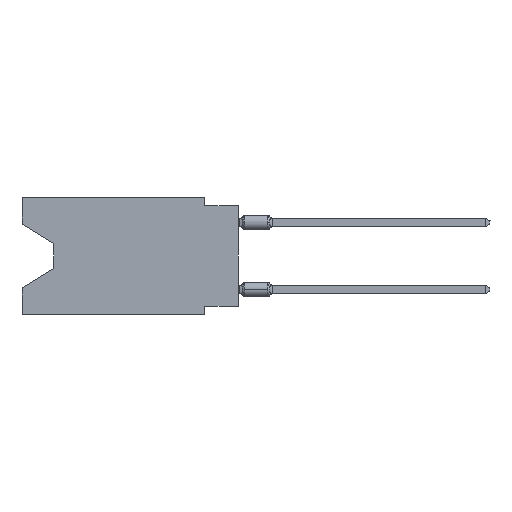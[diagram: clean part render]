
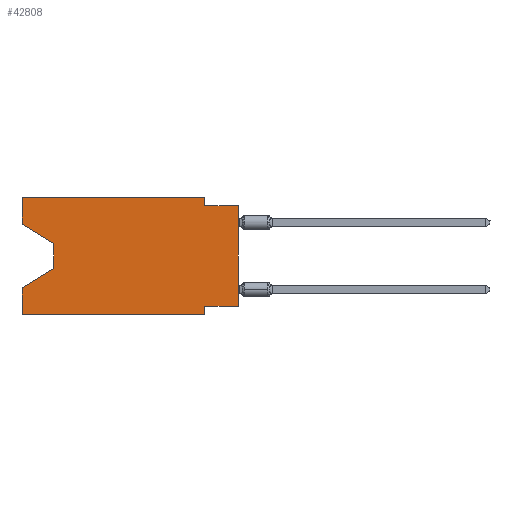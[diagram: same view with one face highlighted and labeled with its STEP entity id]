
A CAD part, left-side view. The second image highlights one B-rep face of the part: STEP entity #42808.
In plain terms, the highlighted planar face has unit normal (-1, 0, 0).
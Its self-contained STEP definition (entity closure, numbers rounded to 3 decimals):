
#393 = VECTOR ( 'NONE', #52997, 1000. ) ;
#806 = VERTEX_POINT ( 'NONE', #63319 ) ;
#818 = DIRECTION ( 'NONE',  ( 0., -1., 0. ) ) ;
#3317 = CARTESIAN_POINT ( 'NONE',  ( 0., 16.383, 0. ) ) ;
#4105 = EDGE_CURVE ( 'NONE', #806, #37848, #15259, .T. ) ;
#4121 = VERTEX_POINT ( 'NONE', #20977 ) ;
#6021 = CARTESIAN_POINT ( 'NONE',  ( 0., 2.54, -8.89 ) ) ;
#6137 = EDGE_CURVE ( 'NONE', #69450, #10985, #16919, .T. ) ;
#6158 = PLANE ( 'NONE',  #10852 ) ;
#6751 = VECTOR ( 'NONE', #17231, 1000. ) ;
#7241 = DIRECTION ( 'NONE',  ( 0., 0.855, -0.519 ) ) ;
#9700 = CARTESIAN_POINT ( 'NONE',  ( 0., 2.54, -0.635 ) ) ;
#9800 = DIRECTION ( 'NONE',  ( 0., -1., 0. ) ) ;
#10821 = VECTOR ( 'NONE', #56934, 1000. ) ;
#10852 = AXIS2_PLACEMENT_3D ( 'NONE', #21896, #70353, #21548 ) ;
#10985 = VERTEX_POINT ( 'NONE', #53490 ) ;
#12302 = EDGE_CURVE ( 'NONE', #4121, #63209, #33869, .T. ) ;
#13230 = VECTOR ( 'NONE', #44570, 1000. ) ;
#13774 = LINE ( 'NONE', #46919, #10821 ) ;
#13959 = VERTEX_POINT ( 'NONE', #39909 ) ;
#14126 = VERTEX_POINT ( 'NONE', #68708 ) ;
#14382 = EDGE_CURVE ( 'NONE', #14126, #55716, #55510, .T. ) ;
#15259 = LINE ( 'NONE', #42722, #27439 ) ;
#16164 = LINE ( 'NONE', #59671, #6751 ) ;
#16919 = LINE ( 'NONE', #38690, #42209 ) ;
#17231 = DIRECTION ( 'NONE',  ( 0., 0., -1. ) ) ;
#20310 = CARTESIAN_POINT ( 'NONE',  ( 0., 2.54, 0. ) ) ;
#20862 = CARTESIAN_POINT ( 'NONE',  ( 0., 16.383, 0. ) ) ;
#20977 = CARTESIAN_POINT ( 'NONE',  ( 0., 2.54, -8.255 ) ) ;
#21548 = DIRECTION ( 'NONE',  ( 0., 0., -1. ) ) ;
#21896 = CARTESIAN_POINT ( 'NONE',  ( 0., 16.383, 0. ) ) ;
#22437 = ORIENTED_EDGE ( 'NONE', *, *, #58329, .T. ) ;
#22937 = ORIENTED_EDGE ( 'NONE', *, *, #55519, .F. ) ;
#23330 = CARTESIAN_POINT ( 'NONE',  ( 0., 13.97, -5.385 ) ) ;
#23611 = ORIENTED_EDGE ( 'NONE', *, *, #39152, .F. ) ;
#26426 = EDGE_CURVE ( 'NONE', #37848, #55716, #40421, .T. ) ;
#26533 = FACE_OUTER_BOUND ( 'NONE', #32036, .T. ) ;
#27054 = DIRECTION ( 'NONE',  ( 0., 0., -1. ) ) ;
#27439 = VECTOR ( 'NONE', #27054, 1000. ) ;
#27983 = LINE ( 'NONE', #43311, #67640 ) ;
#28960 = ORIENTED_EDGE ( 'NONE', *, *, #26426, .T. ) ;
#31087 = EDGE_CURVE ( 'NONE', #13959, #806, #68355, .T. ) ;
#32036 = EDGE_LOOP ( 'NONE', ( #70329, #40375, #28960, #38474, #22437, #48964, #60519, #46093, #22937, #23611, #59856, #41739 ) ) ;
#33869 = LINE ( 'NONE', #6021, #13230 ) ;
#33968 = VECTOR ( 'NONE', #57380, 1000. ) ;
#35635 = LINE ( 'NONE', #47025, #33968 ) ;
#36208 = EDGE_CURVE ( 'NONE', #13959, #60650, #35635, .T. ) ;
#36211 = LINE ( 'NONE', #37276, #50064 ) ;
#36373 = VECTOR ( 'NONE', #7241, 1000. ) ;
#37276 = CARTESIAN_POINT ( 'NONE',  ( 0., 0., -8.255 ) ) ;
#37848 = VERTEX_POINT ( 'NONE', #43271 ) ;
#38474 = ORIENTED_EDGE ( 'NONE', *, *, #14382, .F. ) ;
#38690 = CARTESIAN_POINT ( 'NONE',  ( 0., 0., 0. ) ) ;
#39152 = EDGE_CURVE ( 'NONE', #65937, #67887, #16164, .T. ) ;
#39909 = CARTESIAN_POINT ( 'NONE',  ( 0., 16.383, -2.038 ) ) ;
#40375 = ORIENTED_EDGE ( 'NONE', *, *, #4105, .T. ) ;
#40421 = LINE ( 'NONE', #23330, #36373 ) ;
#41035 = VECTOR ( 'NONE', #9800, 1000. ) ;
#41739 = ORIENTED_EDGE ( 'NONE', *, *, #36208, .F. ) ;
#42209 = VECTOR ( 'NONE', #54005, 1000. ) ;
#42265 = DIRECTION ( 'NONE',  ( 0., 1., 0. ) ) ;
#42722 = CARTESIAN_POINT ( 'NONE',  ( 0., 13.97, -3.505 ) ) ;
#42808 = ADVANCED_FACE ( 'NONE', ( #26533 ), #6158, .F. ) ;
#43271 = CARTESIAN_POINT ( 'NONE',  ( 0., 13.97, -5.385 ) ) ;
#43311 = CARTESIAN_POINT ( 'NONE',  ( 0., 0., -0.635 ) ) ;
#43753 = CARTESIAN_POINT ( 'NONE',  ( 0., 16.383, 0. ) ) ;
#44570 = DIRECTION ( 'NONE',  ( 0., 0., -1. ) ) ;
#45770 = CARTESIAN_POINT ( 'NONE',  ( 0., 16.383, -6.852 ) ) ;
#46093 = ORIENTED_EDGE ( 'NONE', *, *, #6137, .T. ) ;
#46284 = CARTESIAN_POINT ( 'NONE',  ( 0., 2.54, -8.89 ) ) ;
#46919 = CARTESIAN_POINT ( 'NONE',  ( 0., 16.383, -8.89 ) ) ;
#47025 = CARTESIAN_POINT ( 'NONE',  ( 0., 16.383, 0. ) ) ;
#48024 = EDGE_CURVE ( 'NONE', #69450, #4121, #36211, .T. ) ;
#48964 = ORIENTED_EDGE ( 'NONE', *, *, #12302, .F. ) ;
#50064 = VECTOR ( 'NONE', #42265, 1000. ) ;
#52997 = DIRECTION ( 'NONE',  ( 0., -0.855, -0.519 ) ) ;
#53490 = CARTESIAN_POINT ( 'NONE',  ( 0., 0., -0.635 ) ) ;
#54005 = DIRECTION ( 'NONE',  ( 0., 0., 1. ) ) ;
#54013 = LINE ( 'NONE', #20862, #41035 ) ;
#55510 = LINE ( 'NONE', #43753, #67239 ) ;
#55519 = EDGE_CURVE ( 'NONE', #67887, #10985, #27983, .T. ) ;
#55716 = VERTEX_POINT ( 'NONE', #45770 ) ;
#56934 = DIRECTION ( 'NONE',  ( 0., -1., 0. ) ) ;
#57380 = DIRECTION ( 'NONE',  ( 0., 0., 1. ) ) ;
#58329 = EDGE_CURVE ( 'NONE', #14126, #63209, #13774, .T. ) ;
#59671 = CARTESIAN_POINT ( 'NONE',  ( 0., 2.54, 0. ) ) ;
#59856 = ORIENTED_EDGE ( 'NONE', *, *, #68648, .F. ) ;
#60519 = ORIENTED_EDGE ( 'NONE', *, *, #48024, .F. ) ;
#60650 = VERTEX_POINT ( 'NONE', #3317 ) ;
#61218 = DIRECTION ( 'NONE',  ( 0., 0., 1. ) ) ;
#63209 = VERTEX_POINT ( 'NONE', #46284 ) ;
#63319 = CARTESIAN_POINT ( 'NONE',  ( 0., 13.97, -3.505 ) ) ;
#64538 = CARTESIAN_POINT ( 'NONE',  ( 0., 0., -8.255 ) ) ;
#65937 = VERTEX_POINT ( 'NONE', #20310 ) ;
#67239 = VECTOR ( 'NONE', #61218, 1000. ) ;
#67640 = VECTOR ( 'NONE', #818, 1000. ) ;
#67887 = VERTEX_POINT ( 'NONE', #9700 ) ;
#68355 = LINE ( 'NONE', #68685, #393 ) ;
#68648 = EDGE_CURVE ( 'NONE', #60650, #65937, #54013, .T. ) ;
#68685 = CARTESIAN_POINT ( 'NONE',  ( 0., 16.383, -2.038 ) ) ;
#68708 = CARTESIAN_POINT ( 'NONE',  ( 0., 16.383, -8.89 ) ) ;
#69450 = VERTEX_POINT ( 'NONE', #64538 ) ;
#70329 = ORIENTED_EDGE ( 'NONE', *, *, #31087, .T. ) ;
#70353 = DIRECTION ( 'NONE',  ( 1., 0., 0. ) ) ;
